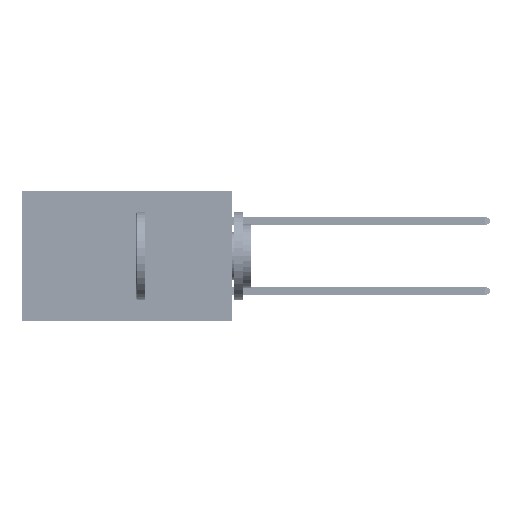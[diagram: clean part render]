
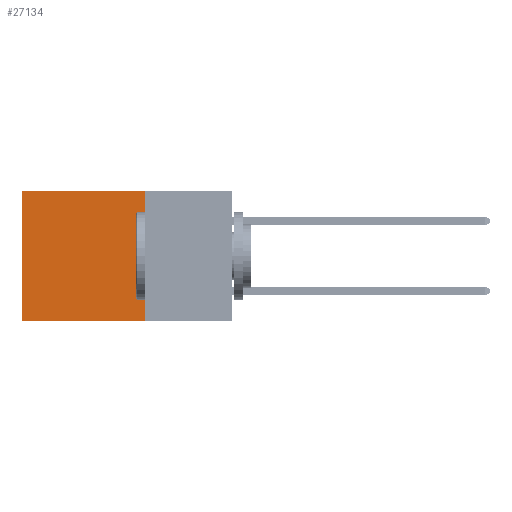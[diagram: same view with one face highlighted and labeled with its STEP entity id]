
A CAD part, left-side view. The second image highlights one B-rep face of the part: STEP entity #27134.
In plain terms, the highlighted planar face has unit normal (-1, 0, 0).
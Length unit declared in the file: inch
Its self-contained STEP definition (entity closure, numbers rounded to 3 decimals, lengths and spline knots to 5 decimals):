
#444 = EDGE_CURVE ( 'NONE', #32138, #47345, #18604, .T. ) ;
#498 = ORIENTED_EDGE ( 'NONE', *, *, #49013, .F. ) ;
#1243 = CARTESIAN_POINT ( 'NONE',  ( 0.2875, 0.6, 0. ) ) ;
#2471 = CARTESIAN_POINT ( 'NONE',  ( 0.2875, 0.6, 0. ) ) ;
#3540 = LINE ( 'NONE', #11744, #15120 ) ;
#5150 = PLANE ( 'NONE',  #46642 ) ;
#6392 = CARTESIAN_POINT ( 'NONE',  ( 0.2875, 0.25, 0. ) ) ;
#7755 = ORIENTED_EDGE ( 'NONE', *, *, #444, .T. ) ;
#10043 = DIRECTION ( 'NONE',  ( 0., 0., -1. ) ) ;
#10115 = EDGE_LOOP ( 'NONE', ( #7755, #16296, #498, #49872 ) ) ;
#10698 = EDGE_CURVE ( 'NONE', #41118, #47345, #3540, .T. ) ;
#11744 = CARTESIAN_POINT ( 'NONE',  ( 0.2875, 0.25, -0.37 ) ) ;
#13088 = VECTOR ( 'NONE', #10043, 39.37008 ) ;
#13454 = LINE ( 'NONE', #6392, #47581 ) ;
#14565 = CARTESIAN_POINT ( 'NONE',  ( 0.2875, 0.6, -0.37 ) ) ;
#15120 = VECTOR ( 'NONE', #42406, 39.37008 ) ;
#15669 = EDGE_CURVE ( 'NONE', #33999, #32138, #50018, .T. ) ;
#16296 = ORIENTED_EDGE ( 'NONE', *, *, #10698, .F. ) ;
#18604 = LINE ( 'NONE', #2471, #13088 ) ;
#23847 = VECTOR ( 'NONE', #49890, 39.37008 ) ;
#25917 = FACE_OUTER_BOUND ( 'NONE', #10115, .T. ) ;
#27134 = ADVANCED_FACE ( 'NONE', ( #25917 ), #5150, .F. ) ;
#27562 = CARTESIAN_POINT ( 'NONE',  ( 0.2875, 0.25, -0.37 ) ) ;
#30627 = CARTESIAN_POINT ( 'NONE',  ( 0.2875, 0.25, 0. ) ) ;
#32138 = VERTEX_POINT ( 'NONE', #1243 ) ;
#32306 = DIRECTION ( 'NONE',  ( 0., 0., -1. ) ) ;
#33573 = DIRECTION ( 'NONE',  ( 0., 0., -1. ) ) ;
#33999 = VERTEX_POINT ( 'NONE', #48820 ) ;
#41118 = VERTEX_POINT ( 'NONE', #27562 ) ;
#42406 = DIRECTION ( 'NONE',  ( 0., 1., 0. ) ) ;
#44407 = DIRECTION ( 'NONE',  ( 1., 0., 0. ) ) ;
#46642 = AXIS2_PLACEMENT_3D ( 'NONE', #48501, #44407, #32306 ) ;
#47345 = VERTEX_POINT ( 'NONE', #14565 ) ;
#47581 = VECTOR ( 'NONE', #33573, 39.37008 ) ;
#48501 = CARTESIAN_POINT ( 'NONE',  ( 0.2875, 0.25, 0. ) ) ;
#48820 = CARTESIAN_POINT ( 'NONE',  ( 0.2875, 0.25, 0. ) ) ;
#49013 = EDGE_CURVE ( 'NONE', #33999, #41118, #13454, .T. ) ;
#49872 = ORIENTED_EDGE ( 'NONE', *, *, #15669, .T. ) ;
#49890 = DIRECTION ( 'NONE',  ( 0., 1., 0. ) ) ;
#50018 = LINE ( 'NONE', #30627, #23847 ) ;
